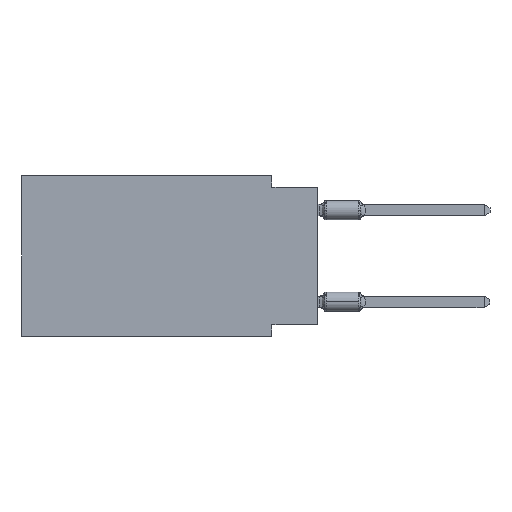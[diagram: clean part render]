
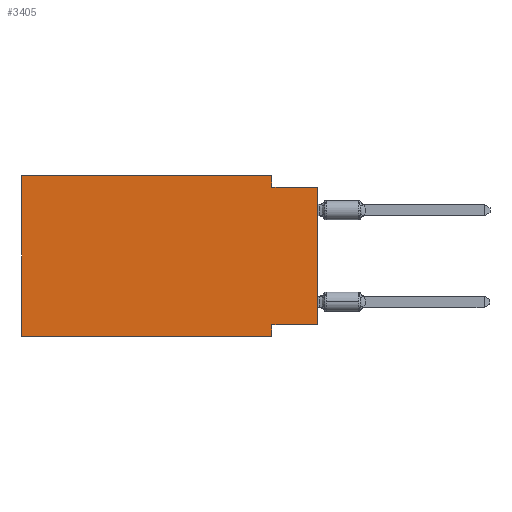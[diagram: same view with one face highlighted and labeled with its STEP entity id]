
A CAD part, left-side view. The second image highlights one B-rep face of the part: STEP entity #3405.
In plain terms, the highlighted planar face has unit normal (-1, 0, 0).
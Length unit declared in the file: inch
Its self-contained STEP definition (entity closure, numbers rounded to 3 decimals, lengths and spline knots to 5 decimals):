
#131 = VECTOR ( 'NONE', #12263, 39.37008 ) ;
#326 = EDGE_CURVE ( 'NONE', #14025, #6365, #13071, .T. ) ;
#347 = DIRECTION ( 'NONE',  ( 0., 0., -1. ) ) ;
#381 = CARTESIAN_POINT ( 'NONE',  ( 0., 0., 0. ) ) ;
#1592 = CARTESIAN_POINT ( 'NONE',  ( 0., 0.1, 0. ) ) ;
#1640 = DIRECTION ( 'NONE',  ( 0., -1., 0. ) ) ;
#1893 = VECTOR ( 'NONE', #8298, 39.37008 ) ;
#2172 = VECTOR ( 'NONE', #12060, 39.37008 ) ;
#2491 = EDGE_CURVE ( 'NONE', #11022, #6170, #8909, .T. ) ;
#2667 = CARTESIAN_POINT ( 'NONE',  ( 0., 0.1, -0.35 ) ) ;
#3391 = DIRECTION ( 'NONE',  ( 0., -1., 0. ) ) ;
#3405 = ADVANCED_FACE ( 'NONE', ( #7633 ), #4177, .F. ) ;
#3635 = DIRECTION ( 'NONE',  ( 0., 1., 0. ) ) ;
#3678 = VECTOR ( 'NONE', #3635, 39.37008 ) ;
#3686 = ORIENTED_EDGE ( 'NONE', *, *, #2491, .F. ) ;
#4063 = ORIENTED_EDGE ( 'NONE', *, *, #6209, .T. ) ;
#4177 = PLANE ( 'NONE',  #6277 ) ;
#4295 = EDGE_CURVE ( 'NONE', #10654, #11022, #12293, .T. ) ;
#4761 = CARTESIAN_POINT ( 'NONE',  ( 0., 0.1, 0. ) ) ;
#5094 = LINE ( 'NONE', #13205, #11247 ) ;
#5421 = VERTEX_POINT ( 'NONE', #7988 ) ;
#5548 = DIRECTION ( 'NONE',  ( 0., 0., -1. ) ) ;
#5549 = VERTEX_POINT ( 'NONE', #14586 ) ;
#5882 = EDGE_CURVE ( 'NONE', #11552, #5421, #5094, .T. ) ;
#6170 = VERTEX_POINT ( 'NONE', #11641 ) ;
#6209 = EDGE_CURVE ( 'NONE', #11552, #6365, #9621, .T. ) ;
#6277 = AXIS2_PLACEMENT_3D ( 'NONE', #8860, #13589, #5548 ) ;
#6365 = VERTEX_POINT ( 'NONE', #12490 ) ;
#7633 = FACE_OUTER_BOUND ( 'NONE', #10911, .T. ) ;
#7917 = CARTESIAN_POINT ( 'NONE',  ( 0., 0.645, -0.35 ) ) ;
#7988 = CARTESIAN_POINT ( 'NONE',  ( 0., 0.645, 0. ) ) ;
#8021 = CARTESIAN_POINT ( 'NONE',  ( 0., 0., -0.325 ) ) ;
#8043 = VECTOR ( 'NONE', #347, 39.37008 ) ;
#8298 = DIRECTION ( 'NONE',  ( 0., 0., 1. ) ) ;
#8510 = VECTOR ( 'NONE', #1640, 39.37008 ) ;
#8860 = CARTESIAN_POINT ( 'NONE',  ( 0., 0.645, 0. ) ) ;
#8909 = LINE ( 'NONE', #14547, #131 ) ;
#9001 = VECTOR ( 'NONE', #3391, 39.37008 ) ;
#9131 = CARTESIAN_POINT ( 'NONE',  ( 0., 0.1, -0.025 ) ) ;
#9375 = LINE ( 'NONE', #14083, #9001 ) ;
#9621 = LINE ( 'NONE', #14317, #8510 ) ;
#10229 = EDGE_CURVE ( 'NONE', #5549, #14025, #10489, .T. ) ;
#10242 = ORIENTED_EDGE ( 'NONE', *, *, #326, .F. ) ;
#10489 = LINE ( 'NONE', #8021, #3678 ) ;
#10654 = VERTEX_POINT ( 'NONE', #4761 ) ;
#10911 = EDGE_LOOP ( 'NONE', ( #14278, #3686, #13292, #12122, #11982, #4063, #10242, #15073 ) ) ;
#11022 = VERTEX_POINT ( 'NONE', #9131 ) ;
#11247 = VECTOR ( 'NONE', #13513, 39.37008 ) ;
#11552 = VERTEX_POINT ( 'NONE', #7917 ) ;
#11589 = EDGE_CURVE ( 'NONE', #5421, #10654, #9375, .T. ) ;
#11641 = CARTESIAN_POINT ( 'NONE',  ( 0., 0., -0.025 ) ) ;
#11737 = EDGE_CURVE ( 'NONE', #5549, #6170, #14165, .T. ) ;
#11982 = ORIENTED_EDGE ( 'NONE', *, *, #5882, .F. ) ;
#12060 = DIRECTION ( 'NONE',  ( 0., 0., -1. ) ) ;
#12122 = ORIENTED_EDGE ( 'NONE', *, *, #11589, .F. ) ;
#12263 = DIRECTION ( 'NONE',  ( 0., -1., 0. ) ) ;
#12293 = LINE ( 'NONE', #1592, #8043 ) ;
#12490 = CARTESIAN_POINT ( 'NONE',  ( 0., 0.1, -0.35 ) ) ;
#13071 = LINE ( 'NONE', #2667, #2172 ) ;
#13205 = CARTESIAN_POINT ( 'NONE',  ( 0., 0.645, 0. ) ) ;
#13292 = ORIENTED_EDGE ( 'NONE', *, *, #4295, .F. ) ;
#13513 = DIRECTION ( 'NONE',  ( 0., 0., 1. ) ) ;
#13589 = DIRECTION ( 'NONE',  ( 1., 0., 0. ) ) ;
#14025 = VERTEX_POINT ( 'NONE', #14577 ) ;
#14083 = CARTESIAN_POINT ( 'NONE',  ( 0., 0.645, 0. ) ) ;
#14165 = LINE ( 'NONE', #381, #1893 ) ;
#14278 = ORIENTED_EDGE ( 'NONE', *, *, #11737, .T. ) ;
#14317 = CARTESIAN_POINT ( 'NONE',  ( 0., 0.645, -0.35 ) ) ;
#14547 = CARTESIAN_POINT ( 'NONE',  ( 0., 0., -0.025 ) ) ;
#14577 = CARTESIAN_POINT ( 'NONE',  ( 0., 0.1, -0.325 ) ) ;
#14586 = CARTESIAN_POINT ( 'NONE',  ( 0., 0., -0.325 ) ) ;
#15073 = ORIENTED_EDGE ( 'NONE', *, *, #10229, .F. ) ;
